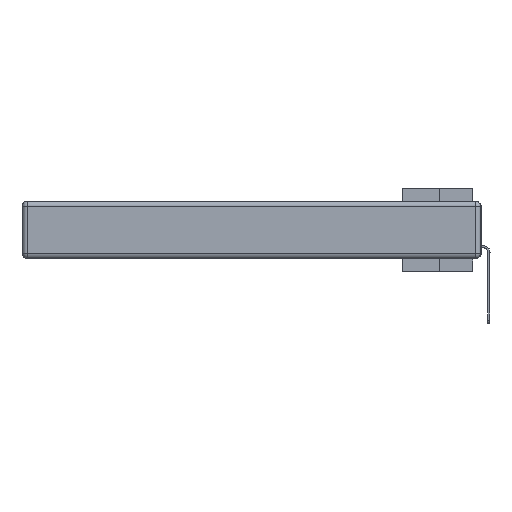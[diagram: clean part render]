
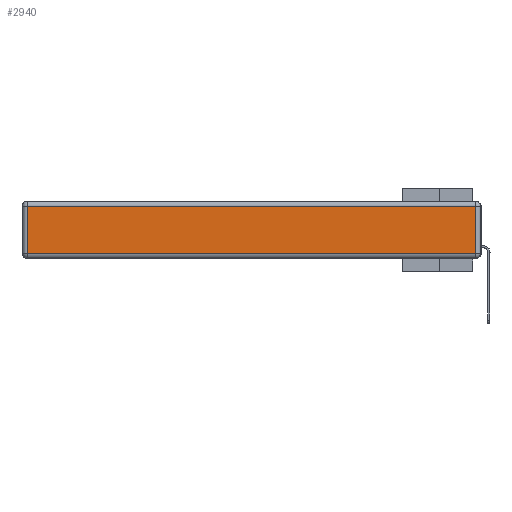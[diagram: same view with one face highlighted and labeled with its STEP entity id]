
A CAD part, left-side view. The second image highlights one B-rep face of the part: STEP entity #2940.
In plain terms, the highlighted planar face has unit normal (-1, 0, 0).
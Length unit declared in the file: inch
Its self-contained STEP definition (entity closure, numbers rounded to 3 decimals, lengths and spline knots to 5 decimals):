
#2150 = ORIENTED_EDGE ( 'NONE', *, *, #2831, .T. ) ;
#2372 = PLANE ( 'NONE',  #27669 ) ;
#2831 = EDGE_CURVE ( 'NONE', #33428, #22927, #39616, .T. ) ;
#2940 = ADVANCED_FACE ( 'NONE', ( #30859 ), #2372, .T. ) ;
#3418 = CARTESIAN_POINT ( 'NONE',  ( 0., 0.03, -0.313 ) ) ;
#5075 = ORIENTED_EDGE ( 'NONE', *, *, #9548, .T. ) ;
#5076 = VECTOR ( 'NONE', #5481, 39.37008 ) ;
#5481 = DIRECTION ( 'NONE',  ( 0., 0., -1. ) ) ;
#5595 = ORIENTED_EDGE ( 'NONE', *, *, #23622, .T. ) ;
#5701 = ORIENTED_EDGE ( 'NONE', *, *, #38604, .T. ) ;
#6439 = CARTESIAN_POINT ( 'NONE',  ( 0., 0.03, -0.03 ) ) ;
#9548 = EDGE_CURVE ( 'NONE', #33639, #33428, #28642, .T. ) ;
#14001 = CARTESIAN_POINT ( 'NONE',  ( 0., 0.03, -0.343 ) ) ;
#15006 = VECTOR ( 'NONE', #36060, 39.37008 ) ;
#15040 = CARTESIAN_POINT ( 'NONE',  ( 0., 0., -0.343 ) ) ;
#17916 = VECTOR ( 'NONE', #40927, 39.37008 ) ;
#20458 = LINE ( 'NONE', #14001, #15006 ) ;
#20771 = EDGE_LOOP ( 'NONE', ( #5595, #5701, #5075, #2150 ) ) ;
#21032 = LINE ( 'NONE', #39960, #38702 ) ;
#21656 = VERTEX_POINT ( 'NONE', #3418 ) ;
#22927 = VERTEX_POINT ( 'NONE', #35252 ) ;
#23622 = EDGE_CURVE ( 'NONE', #22927, #21656, #21032, .T. ) ;
#24359 = DIRECTION ( 'NONE',  ( 0., -1., 0. ) ) ;
#24827 = DIRECTION ( 'NONE',  ( -1., 0., 0. ) ) ;
#27669 = AXIS2_PLACEMENT_3D ( 'NONE', #15040, #24827, #27755 ) ;
#27755 = DIRECTION ( 'NONE',  ( 0., 0., 1. ) ) ;
#28642 = LINE ( 'NONE', #31354, #17916 ) ;
#30595 = CARTESIAN_POINT ( 'NONE',  ( 0., 2.72, -0.03 ) ) ;
#30859 = FACE_OUTER_BOUND ( 'NONE', #20771, .T. ) ;
#31354 = CARTESIAN_POINT ( 'NONE',  ( 0., 2.75, -0.03 ) ) ;
#33428 = VERTEX_POINT ( 'NONE', #30595 ) ;
#33639 = VERTEX_POINT ( 'NONE', #6439 ) ;
#33973 = CARTESIAN_POINT ( 'NONE',  ( 0., 2.72, -0.343 ) ) ;
#35252 = CARTESIAN_POINT ( 'NONE',  ( 0., 2.72, -0.313 ) ) ;
#36060 = DIRECTION ( 'NONE',  ( 0., 0., 1. ) ) ;
#38604 = EDGE_CURVE ( 'NONE', #21656, #33639, #20458, .T. ) ;
#38702 = VECTOR ( 'NONE', #24359, 39.37008 ) ;
#39616 = LINE ( 'NONE', #33973, #5076 ) ;
#39960 = CARTESIAN_POINT ( 'NONE',  ( 0., 0., -0.313 ) ) ;
#40927 = DIRECTION ( 'NONE',  ( 0., 1., 0. ) ) ;
